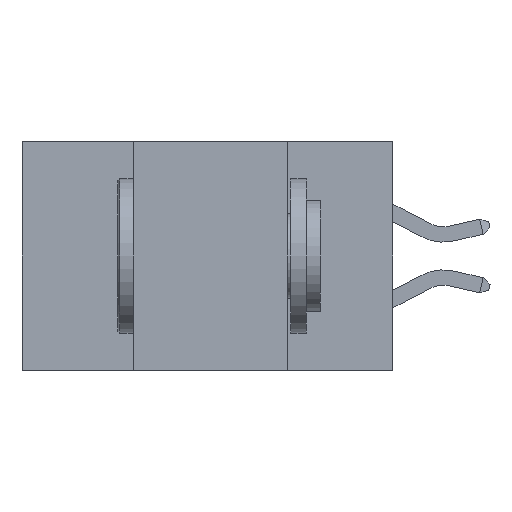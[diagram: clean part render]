
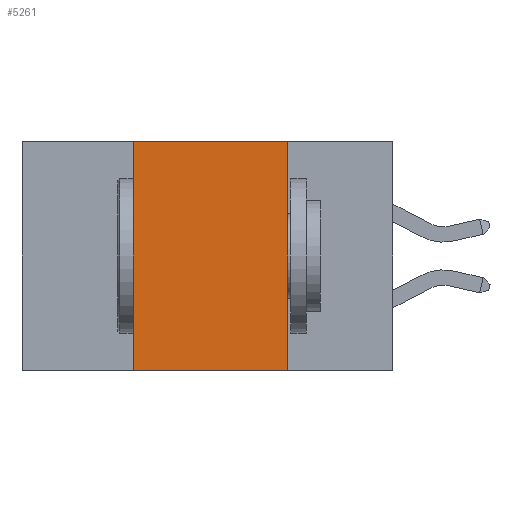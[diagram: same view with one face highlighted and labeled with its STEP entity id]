
A CAD part, left-side view. The second image highlights one B-rep face of the part: STEP entity #5261.
In plain terms, the highlighted planar face has unit normal (-1, 0, 0).
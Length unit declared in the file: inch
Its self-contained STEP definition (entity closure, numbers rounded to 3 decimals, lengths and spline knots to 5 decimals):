
#875 = DIRECTION ( 'NONE',  ( 0., 0., -1. ) ) ;
#3937 = ORIENTED_EDGE ( 'NONE', *, *, #31993, .F. ) ;
#4502 = ORIENTED_EDGE ( 'NONE', *, *, #11961, .F. ) ;
#5261 = ADVANCED_FACE ( 'NONE', ( #31809 ), #40534, .F. ) ;
#5889 = CARTESIAN_POINT ( 'NONE',  ( 0., 0.6, 0. ) ) ;
#5959 = LINE ( 'NONE', #20308, #41856 ) ;
#9340 = DIRECTION ( 'NONE',  ( 0., 0., -1. ) ) ;
#11234 = EDGE_CURVE ( 'NONE', #39438, #32498, #27035, .T. ) ;
#11961 = EDGE_CURVE ( 'NONE', #17901, #26701, #18233, .T. ) ;
#13394 = EDGE_LOOP ( 'NONE', ( #41116, #4502, #3937, #17604 ) ) ;
#17604 = ORIENTED_EDGE ( 'NONE', *, *, #11234, .T. ) ;
#17741 = VECTOR ( 'NONE', #21480, 39.37008 ) ;
#17837 = CARTESIAN_POINT ( 'NONE',  ( 0., 0.6, -0.37 ) ) ;
#17901 = VERTEX_POINT ( 'NONE', #33668 ) ;
#18233 = LINE ( 'NONE', #42352, #44814 ) ;
#20308 = CARTESIAN_POINT ( 'NONE',  ( 0., 0.42, 0. ) ) ;
#21480 = DIRECTION ( 'NONE',  ( 0., -1., 0. ) ) ;
#21752 = CARTESIAN_POINT ( 'NONE',  ( 0., 0.17, 0. ) ) ;
#23448 = CARTESIAN_POINT ( 'NONE',  ( 0., 0.17, 0. ) ) ;
#26116 = AXIS2_PLACEMENT_3D ( 'NONE', #5889, #30311, #9340 ) ;
#26540 = CARTESIAN_POINT ( 'NONE',  ( 0., 0.17, -0.37 ) ) ;
#26701 = VERTEX_POINT ( 'NONE', #23448 ) ;
#27035 = LINE ( 'NONE', #17837, #17741 ) ;
#27072 = EDGE_CURVE ( 'NONE', #26701, #32498, #28770, .T. ) ;
#27507 = DIRECTION ( 'NONE',  ( 0., 0., 1. ) ) ;
#27682 = VECTOR ( 'NONE', #875, 39.37008 ) ;
#27859 = CARTESIAN_POINT ( 'NONE',  ( 0., 0.42, -0.37 ) ) ;
#28770 = LINE ( 'NONE', #21752, #27682 ) ;
#30311 = DIRECTION ( 'NONE',  ( 1., 0., 0. ) ) ;
#31809 = FACE_OUTER_BOUND ( 'NONE', #13394, .T. ) ;
#31993 = EDGE_CURVE ( 'NONE', #39438, #17901, #5959, .T. ) ;
#32498 = VERTEX_POINT ( 'NONE', #26540 ) ;
#33668 = CARTESIAN_POINT ( 'NONE',  ( 0., 0.42, 0. ) ) ;
#35415 = DIRECTION ( 'NONE',  ( 0., -1., 0. ) ) ;
#39438 = VERTEX_POINT ( 'NONE', #27859 ) ;
#40534 = PLANE ( 'NONE',  #26116 ) ;
#41116 = ORIENTED_EDGE ( 'NONE', *, *, #27072, .F. ) ;
#41856 = VECTOR ( 'NONE', #27507, 39.37008 ) ;
#42352 = CARTESIAN_POINT ( 'NONE',  ( 0., 0.6, 0. ) ) ;
#44814 = VECTOR ( 'NONE', #35415, 39.37008 ) ;
